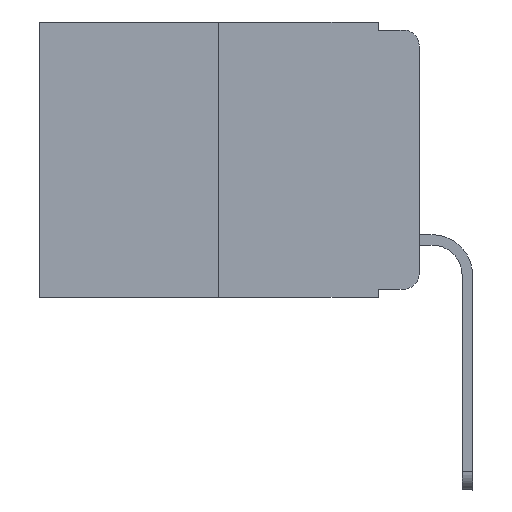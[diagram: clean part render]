
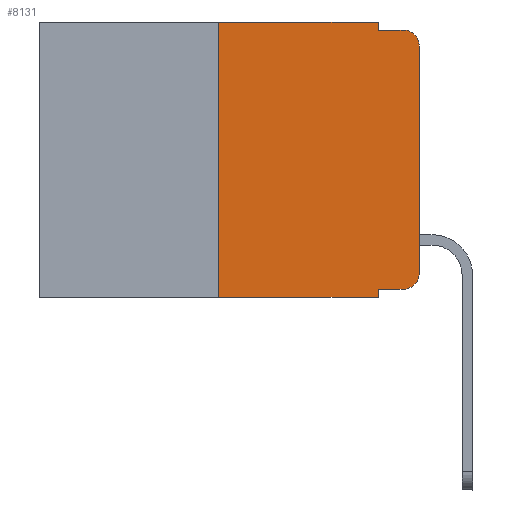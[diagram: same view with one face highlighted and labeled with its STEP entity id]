
A CAD part, left-side view. The second image highlights one B-rep face of the part: STEP entity #8131.
In plain terms, the highlighted planar face has unit normal (-1, 0, 0).
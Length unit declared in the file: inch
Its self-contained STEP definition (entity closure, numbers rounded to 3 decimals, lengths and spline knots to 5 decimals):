
#78 = VECTOR ( 'NONE', #4067, 39.37008 ) ;
#334 = VECTOR ( 'NONE', #16598, 39.37008 ) ;
#336 = VERTEX_POINT ( 'NONE', #4671 ) ;
#361 = LINE ( 'NONE', #11068, #9636 ) ;
#1490 = LINE ( 'NONE', #10688, #78 ) ;
#1507 = VERTEX_POINT ( 'NONE', #15355 ) ;
#1818 = AXIS2_PLACEMENT_3D ( 'NONE', #5320, #10719, #14863 ) ;
#1896 = CARTESIAN_POINT ( 'NONE',  ( 0., 0.051, -0.01 ) ) ;
#1909 = EDGE_CURVE ( 'NONE', #7852, #13940, #4561, .T. ) ;
#2077 = EDGE_CURVE ( 'NONE', #17432, #14618, #8900, .T. ) ;
#2202 = CARTESIAN_POINT ( 'NONE',  ( 0., 0.051, -0.01 ) ) ;
#2977 = VECTOR ( 'NONE', #16658, 39.37008 ) ;
#3076 = FACE_OUTER_BOUND ( 'NONE', #6657, .T. ) ;
#3172 = CARTESIAN_POINT ( 'NONE',  ( 0., 0.473, 0. ) ) ;
#3422 = LINE ( 'NONE', #16511, #6775 ) ;
#3519 = ORIENTED_EDGE ( 'NONE', *, *, #4921, .T. ) ;
#3657 = ORIENTED_EDGE ( 'NONE', *, *, #10140, .T. ) ;
#3707 = ORIENTED_EDGE ( 'NONE', *, *, #7051, .F. ) ;
#4067 = DIRECTION ( 'NONE',  ( 0., 0., -1. ) ) ;
#4386 = VECTOR ( 'NONE', #16831, 39.37008 ) ;
#4561 = LINE ( 'NONE', #1896, #2977 ) ;
#4591 = ORIENTED_EDGE ( 'NONE', *, *, #17064, .T. ) ;
#4671 = CARTESIAN_POINT ( 'NONE',  ( 0., 0.051, -0.343 ) ) ;
#4841 = CARTESIAN_POINT ( 'NONE',  ( 0., 0.25, 0. ) ) ;
#4921 = EDGE_CURVE ( 'NONE', #1507, #10523, #12831, .T. ) ;
#5320 = CARTESIAN_POINT ( 'NONE',  ( 0., 0.02, -0.03 ) ) ;
#5422 = DIRECTION ( 'NONE',  ( 0., -1., 0. ) ) ;
#5683 = DIRECTION ( 'NONE',  ( 0., -1., 0. ) ) ;
#5693 = CIRCLE ( 'NONE', #15859, 0.02 ) ;
#6049 = CARTESIAN_POINT ( 'NONE',  ( 0., 0.051, -0.333 ) ) ;
#6190 = CARTESIAN_POINT ( 'NONE',  ( 0., 0.02, -0.313 ) ) ;
#6422 = CARTESIAN_POINT ( 'NONE',  ( 0., 0.02, -0.01 ) ) ;
#6657 = EDGE_LOOP ( 'NONE', ( #16941, #3657, #16131, #9294, #3707, #9297, #14115, #16953, #3519, #4591 ) ) ;
#6775 = VECTOR ( 'NONE', #12774, 39.37008 ) ;
#7051 = EDGE_CURVE ( 'NONE', #14249, #7623, #361, .T. ) ;
#7062 = DIRECTION ( 'NONE',  ( 1., 0., 0. ) ) ;
#7588 = CARTESIAN_POINT ( 'NONE',  ( 0., 0., -0.313 ) ) ;
#7623 = VERTEX_POINT ( 'NONE', #8595 ) ;
#7852 = VERTEX_POINT ( 'NONE', #2202 ) ;
#8131 = ADVANCED_FACE ( 'NONE', ( #3076 ), #15176, .F. ) ;
#8134 = EDGE_CURVE ( 'NONE', #17299, #336, #8576, .T. ) ;
#8223 = CARTESIAN_POINT ( 'NONE',  ( 0., 0.02, -0.333 ) ) ;
#8576 = LINE ( 'NONE', #13932, #334 ) ;
#8595 = CARTESIAN_POINT ( 'NONE',  ( 0., 0.051, 0. ) ) ;
#8900 = LINE ( 'NONE', #10470, #4386 ) ;
#9002 = DIRECTION ( 'NONE',  ( 0., 0., 1. ) ) ;
#9043 = EDGE_CURVE ( 'NONE', #7623, #7852, #1490, .T. ) ;
#9294 = ORIENTED_EDGE ( 'NONE', *, *, #9043, .F. ) ;
#9297 = ORIENTED_EDGE ( 'NONE', *, *, #16106, .F. ) ;
#9636 = VECTOR ( 'NONE', #5422, 39.37008 ) ;
#10140 = EDGE_CURVE ( 'NONE', #14618, #13940, #17060, .T. ) ;
#10368 = VECTOR ( 'NONE', #5683, 39.37008 ) ;
#10470 = CARTESIAN_POINT ( 'NONE',  ( 0., 0., 0. ) ) ;
#10523 = VERTEX_POINT ( 'NONE', #8223 ) ;
#10688 = CARTESIAN_POINT ( 'NONE',  ( 0., 0.051, 0. ) ) ;
#10719 = DIRECTION ( 'NONE',  ( -1., 0., 0. ) ) ;
#11068 = CARTESIAN_POINT ( 'NONE',  ( 0., 0.473, 0. ) ) ;
#11995 = CARTESIAN_POINT ( 'NONE',  ( 0., 0., -0.03 ) ) ;
#12609 = DIRECTION ( 'NONE',  ( 0., 0., -1. ) ) ;
#12774 = DIRECTION ( 'NONE',  ( 0., 0., -1. ) ) ;
#12831 = LINE ( 'NONE', #6049, #10368 ) ;
#12858 = LINE ( 'NONE', #4841, #17245 ) ;
#13811 = EDGE_CURVE ( 'NONE', #1507, #336, #3422, .T. ) ;
#13928 = CARTESIAN_POINT ( 'NONE',  ( 0., 0.25, -0.343 ) ) ;
#13932 = CARTESIAN_POINT ( 'NONE',  ( 0., 0.473, -0.343 ) ) ;
#13940 = VERTEX_POINT ( 'NONE', #6422 ) ;
#14115 = ORIENTED_EDGE ( 'NONE', *, *, #8134, .T. ) ;
#14165 = AXIS2_PLACEMENT_3D ( 'NONE', #3172, #7062, #12609 ) ;
#14249 = VERTEX_POINT ( 'NONE', #16259 ) ;
#14560 = DIRECTION ( 'NONE',  ( 0., 0., -1. ) ) ;
#14618 = VERTEX_POINT ( 'NONE', #11995 ) ;
#14863 = DIRECTION ( 'NONE',  ( 0., 0., -1. ) ) ;
#15176 = PLANE ( 'NONE',  #14165 ) ;
#15355 = CARTESIAN_POINT ( 'NONE',  ( 0., 0.051, -0.333 ) ) ;
#15859 = AXIS2_PLACEMENT_3D ( 'NONE', #6190, #17223, #14560 ) ;
#16106 = EDGE_CURVE ( 'NONE', #17299, #14249, #12858, .T. ) ;
#16131 = ORIENTED_EDGE ( 'NONE', *, *, #1909, .F. ) ;
#16259 = CARTESIAN_POINT ( 'NONE',  ( 0., 0.25, 0. ) ) ;
#16511 = CARTESIAN_POINT ( 'NONE',  ( 0., 0.051, 0. ) ) ;
#16598 = DIRECTION ( 'NONE',  ( 0., -1., 0. ) ) ;
#16658 = DIRECTION ( 'NONE',  ( 0., -1., 0. ) ) ;
#16831 = DIRECTION ( 'NONE',  ( 0., 0., 1. ) ) ;
#16941 = ORIENTED_EDGE ( 'NONE', *, *, #2077, .T. ) ;
#16953 = ORIENTED_EDGE ( 'NONE', *, *, #13811, .F. ) ;
#17060 = CIRCLE ( 'NONE', #1818, 0.02 ) ;
#17064 = EDGE_CURVE ( 'NONE', #10523, #17432, #5693, .T. ) ;
#17223 = DIRECTION ( 'NONE',  ( -1., 0., 0. ) ) ;
#17245 = VECTOR ( 'NONE', #9002, 39.37008 ) ;
#17299 = VERTEX_POINT ( 'NONE', #13928 ) ;
#17432 = VERTEX_POINT ( 'NONE', #7588 ) ;
